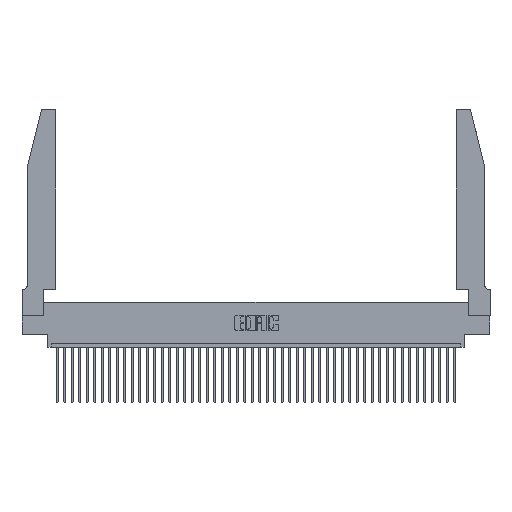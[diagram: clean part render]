
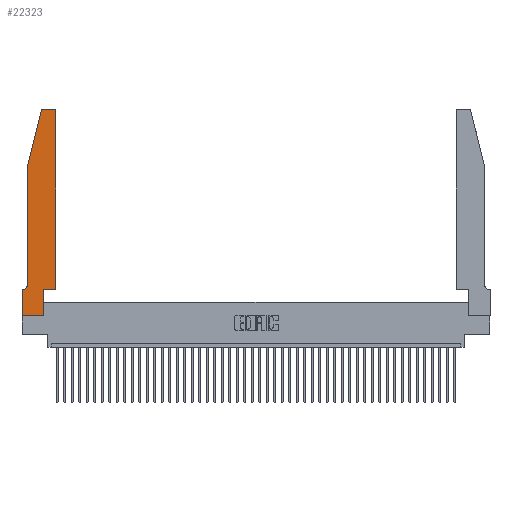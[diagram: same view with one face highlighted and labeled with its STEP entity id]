
A CAD part, top view. The second image highlights one B-rep face of the part: STEP entity #22323.
In plain terms, the highlighted planar face has unit normal (0, 0, 1).
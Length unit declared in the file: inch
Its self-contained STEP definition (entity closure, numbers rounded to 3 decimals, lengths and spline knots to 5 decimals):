
#75 = VECTOR ( 'NONE', #37360, 39.37008 ) ;
#421 = ORIENTED_EDGE ( 'NONE', *, *, #23303, .T. ) ;
#499 = AXIS2_PLACEMENT_3D ( 'NONE', #12375, #32792, #8662 ) ;
#1124 = EDGE_CURVE ( 'NONE', #10636, #11511, #19529, .T. ) ;
#1469 = VECTOR ( 'NONE', #37246, 39.37008 ) ;
#3442 = CARTESIAN_POINT ( 'NONE',  ( 0., 0., 0.37 ) ) ;
#3448 = ORIENTED_EDGE ( 'NONE', *, *, #19866, .T. ) ;
#3503 = VECTOR ( 'NONE', #43739, 39.37008 ) ;
#3626 = ORIENTED_EDGE ( 'NONE', *, *, #1124, .T. ) ;
#3757 = DIRECTION ( 'NONE',  ( -1., 0., 0. ) ) ;
#4185 = EDGE_CURVE ( 'NONE', #25697, #11416, #34772, .T. ) ;
#4944 = CARTESIAN_POINT ( 'NONE',  ( 0., 0., 0.37 ) ) ;
#6909 = CARTESIAN_POINT ( 'NONE',  ( 0.2605, 2.75, 0.37 ) ) ;
#7569 = EDGE_CURVE ( 'NONE', #23483, #25697, #25443, .T. ) ;
#7757 = VECTOR ( 'NONE', #39503, 39.37008 ) ;
#8005 = VECTOR ( 'NONE', #21835, 39.37008 ) ;
#8555 = LINE ( 'NONE', #6909, #43536 ) ;
#8635 = ORIENTED_EDGE ( 'NONE', *, *, #37924, .T. ) ;
#8662 = DIRECTION ( 'NONE',  ( -1., 0., 0. ) ) ;
#8964 = CARTESIAN_POINT ( 'NONE',  ( 0.284, 2.75, 0.37 ) ) ;
#9823 = EDGE_CURVE ( 'NONE', #11739, #15397, #12570, .T. ) ;
#9971 = CARTESIAN_POINT ( 'NONE',  ( 0.25487, 2.72718, 0.37 ) ) ;
#10265 = DIRECTION ( 'NONE',  ( 0., 0., 1. ) ) ;
#10636 = VERTEX_POINT ( 'NONE', #34508 ) ;
#11416 = VERTEX_POINT ( 'NONE', #26267 ) ;
#11511 = VERTEX_POINT ( 'NONE', #26408 ) ;
#11739 = VERTEX_POINT ( 'NONE', #27574 ) ;
#11875 = LINE ( 'NONE', #19484, #38919 ) ;
#12375 = CARTESIAN_POINT ( 'NONE',  ( 0.0055, 0.42, 0.37 ) ) ;
#12570 = LINE ( 'NONE', #30695, #3503 ) ;
#13534 = DIRECTION ( 'NONE',  ( 1., 0., 0. ) ) ;
#15397 = VERTEX_POINT ( 'NONE', #40495 ) ;
#17906 = EDGE_CURVE ( 'NONE', #42066, #19016, #40641, .T. ) ;
#18224 = ORIENTED_EDGE ( 'NONE', *, *, #17906, .T. ) ;
#19016 = VERTEX_POINT ( 'NONE', #35564 ) ;
#19183 = CARTESIAN_POINT ( 'NONE',  ( 0.0755, 2., 0.37 ) ) ;
#19209 = LINE ( 'NONE', #34404, #75 ) ;
#19484 = CARTESIAN_POINT ( 'NONE',  ( 0.0755, 2., 0.37 ) ) ;
#19529 = LINE ( 'NONE', #3442, #1469 ) ;
#19866 = EDGE_CURVE ( 'NONE', #11416, #33592, #36748, .T. ) ;
#20137 = DIRECTION ( 'NONE',  ( 0., 0., 1. ) ) ;
#20427 = CARTESIAN_POINT ( 'NONE',  ( 0., 0.35, 0.37 ) ) ;
#20514 = DIRECTION ( 'NONE',  ( -1., 0., 0. ) ) ;
#20557 = EDGE_CURVE ( 'NONE', #15397, #42066, #19209, .T. ) ;
#20713 = CARTESIAN_POINT ( 'NONE',  ( 0.0755, 2., 0.37 ) ) ;
#20810 = AXIS2_PLACEMENT_3D ( 'NONE', #20427, #20137, #23845 ) ;
#21546 = EDGE_CURVE ( 'NONE', #27714, #38480, #34001, .T. ) ;
#21835 = DIRECTION ( 'NONE',  ( 0., -1., 0. ) ) ;
#22193 = CARTESIAN_POINT ( 'NONE',  ( 0.0755, 0.42, 0.37 ) ) ;
#22264 = ORIENTED_EDGE ( 'NONE', *, *, #9823, .T. ) ;
#22323 = ADVANCED_FACE ( 'NONE', ( #41336 ), #25331, .T. ) ;
#22764 = AXIS2_PLACEMENT_3D ( 'NONE', #29837, #10265, #13534 ) ;
#23303 = EDGE_CURVE ( 'NONE', #33592, #10636, #29215, .T. ) ;
#23319 = ORIENTED_EDGE ( 'NONE', *, *, #7569, .T. ) ;
#23483 = VERTEX_POINT ( 'NONE', #19183 ) ;
#23845 = DIRECTION ( 'NONE',  ( 1., 0., 0. ) ) ;
#24210 = LINE ( 'NONE', #39785, #7757 ) ;
#25331 = PLANE ( 'NONE',  #20810 ) ;
#25443 = LINE ( 'NONE', #20713, #38684 ) ;
#25697 = VERTEX_POINT ( 'NONE', #22193 ) ;
#26267 = CARTESIAN_POINT ( 'NONE',  ( 0.0055, 0.35, 0.37 ) ) ;
#26273 = CARTESIAN_POINT ( 'NONE',  ( 0., 0.35, 0.37 ) ) ;
#26408 = CARTESIAN_POINT ( 'NONE',  ( 0.2865, 0., 0.37 ) ) ;
#27279 = AXIS2_PLACEMENT_3D ( 'NONE', #33639, #37179, #36759 ) ;
#27574 = CARTESIAN_POINT ( 'NONE',  ( 0.2865, 0.35, 0.37 ) ) ;
#27714 = VERTEX_POINT ( 'NONE', #8964 ) ;
#29215 = LINE ( 'NONE', #4944, #8005 ) ;
#29301 = VECTOR ( 'NONE', #3757, 39.37008 ) ;
#29837 = CARTESIAN_POINT ( 'NONE',  ( 0.284, 2.72, 0.37 ) ) ;
#30515 = CARTESIAN_POINT ( 'NONE',  ( 0.4505, 2.72, 0.37 ) ) ;
#30695 = CARTESIAN_POINT ( 'NONE',  ( 0.4505, 0.35, 0.37 ) ) ;
#31418 = ORIENTED_EDGE ( 'NONE', *, *, #41206, .T. ) ;
#32792 = DIRECTION ( 'NONE',  ( 0., 0., -1. ) ) ;
#33592 = VERTEX_POINT ( 'NONE', #26273 ) ;
#33639 = CARTESIAN_POINT ( 'NONE',  ( 0.4205, 2.72, 0.37 ) ) ;
#34001 = CIRCLE ( 'NONE', #22764, 0.03 ) ;
#34404 = CARTESIAN_POINT ( 'NONE',  ( 0.4505, 0.35, 0.37 ) ) ;
#34508 = CARTESIAN_POINT ( 'NONE',  ( 0., 0., 0.37 ) ) ;
#34662 = DIRECTION ( 'NONE',  ( 0., -1., 0. ) ) ;
#34772 = CIRCLE ( 'NONE', #499, 0.07 ) ;
#35564 = CARTESIAN_POINT ( 'NONE',  ( 0.4205, 2.75, 0.37 ) ) ;
#36518 = EDGE_CURVE ( 'NONE', #38480, #23483, #11875, .T. ) ;
#36748 = LINE ( 'NONE', #43787, #29301 ) ;
#36759 = DIRECTION ( 'NONE',  ( 1., 0., 0. ) ) ;
#37179 = DIRECTION ( 'NONE',  ( 0., 0., 1. ) ) ;
#37246 = DIRECTION ( 'NONE',  ( 1., 0., 0. ) ) ;
#37360 = DIRECTION ( 'NONE',  ( 0., 1., 0. ) ) ;
#37924 = EDGE_CURVE ( 'NONE', #19016, #27714, #8555, .T. ) ;
#38480 = VERTEX_POINT ( 'NONE', #9971 ) ;
#38684 = VECTOR ( 'NONE', #34662, 39.37008 ) ;
#38880 = EDGE_LOOP ( 'NONE', ( #8635, #42764, #42915, #23319, #41978, #3448, #421, #3626, #31418, #22264, #42383, #18224 ) ) ;
#38919 = VECTOR ( 'NONE', #43171, 39.37008 ) ;
#39503 = DIRECTION ( 'NONE',  ( 0., 1., 0. ) ) ;
#39785 = CARTESIAN_POINT ( 'NONE',  ( 0.2865, 0.35, 0.37 ) ) ;
#40495 = CARTESIAN_POINT ( 'NONE',  ( 0.4505, 0.35, 0.37 ) ) ;
#40641 = CIRCLE ( 'NONE', #27279, 0.03 ) ;
#41206 = EDGE_CURVE ( 'NONE', #11511, #11739, #24210, .T. ) ;
#41336 = FACE_OUTER_BOUND ( 'NONE', #38880, .T. ) ;
#41978 = ORIENTED_EDGE ( 'NONE', *, *, #4185, .T. ) ;
#42066 = VERTEX_POINT ( 'NONE', #30515 ) ;
#42383 = ORIENTED_EDGE ( 'NONE', *, *, #20557, .T. ) ;
#42764 = ORIENTED_EDGE ( 'NONE', *, *, #21546, .T. ) ;
#42915 = ORIENTED_EDGE ( 'NONE', *, *, #36518, .T. ) ;
#43171 = DIRECTION ( 'NONE',  ( -0.239, -0.971, 0. ) ) ;
#43536 = VECTOR ( 'NONE', #20514, 39.37008 ) ;
#43739 = DIRECTION ( 'NONE',  ( 1., 0., 0. ) ) ;
#43787 = CARTESIAN_POINT ( 'NONE',  ( 0.0755, 0.35, 0.37 ) ) ;
